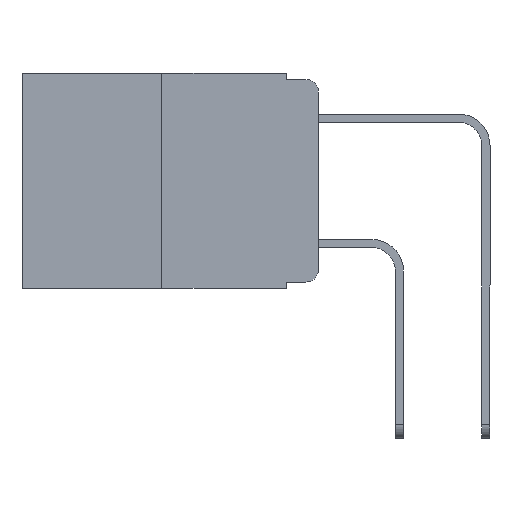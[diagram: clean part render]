
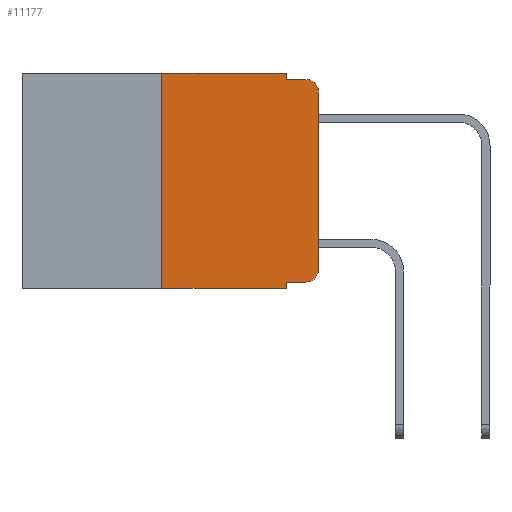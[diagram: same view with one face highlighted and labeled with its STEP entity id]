
A CAD part, left-side view. The second image highlights one B-rep face of the part: STEP entity #11177.
In plain terms, the highlighted planar face has unit normal (-1, 0, 0).
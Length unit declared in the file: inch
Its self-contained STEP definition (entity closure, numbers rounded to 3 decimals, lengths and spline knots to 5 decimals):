
#42 = VERTEX_POINT ( 'NONE', #2022 ) ;
#273 = CARTESIAN_POINT ( 'NONE',  ( 0., 0., 0. ) ) ;
#367 = LINE ( 'NONE', #6275, #9779 ) ;
#527 = CARTESIAN_POINT ( 'NONE',  ( 0., 0.02, -0.01 ) ) ;
#575 = VECTOR ( 'NONE', #2385, 39.37008 ) ;
#760 = CIRCLE ( 'NONE', #11905, 0.02 ) ;
#951 = VERTEX_POINT ( 'NONE', #1294 ) ;
#1268 = CARTESIAN_POINT ( 'NONE',  ( 0., 0.051, -0.333 ) ) ;
#1294 = CARTESIAN_POINT ( 'NONE',  ( 0., 0.25, -0.343 ) ) ;
#1402 = ORIENTED_EDGE ( 'NONE', *, *, #9388, .T. ) ;
#1609 = AXIS2_PLACEMENT_3D ( 'NONE', #4874, #11121, #5756 ) ;
#1796 = CARTESIAN_POINT ( 'NONE',  ( 0., 0., -0.313 ) ) ;
#1931 = ORIENTED_EDGE ( 'NONE', *, *, #2397, .T. ) ;
#1970 = CARTESIAN_POINT ( 'NONE',  ( 0., 0.473, 0. ) ) ;
#2022 = CARTESIAN_POINT ( 'NONE',  ( 0., 0.051, -0.01 ) ) ;
#2036 = LINE ( 'NONE', #2181, #11490 ) ;
#2161 = VERTEX_POINT ( 'NONE', #1268 ) ;
#2181 = CARTESIAN_POINT ( 'NONE',  ( 0., 0.051, -0.333 ) ) ;
#2385 = DIRECTION ( 'NONE',  ( 0., 0., 1. ) ) ;
#2397 = EDGE_CURVE ( 'NONE', #2161, #5680, #2036, .T. ) ;
#2660 = DIRECTION ( 'NONE',  ( 0., 0., -1. ) ) ;
#2750 = CARTESIAN_POINT ( 'NONE',  ( 0., 0.25, 0. ) ) ;
#2762 = CARTESIAN_POINT ( 'NONE',  ( 0., 0.051, -0.01 ) ) ;
#2780 = DIRECTION ( 'NONE',  ( 0., -1., 0. ) ) ;
#2800 = ORIENTED_EDGE ( 'NONE', *, *, #3113, .F. ) ;
#2962 = DIRECTION ( 'NONE',  ( 0., -1., 0. ) ) ;
#3113 = EDGE_CURVE ( 'NONE', #42, #8271, #11598, .T. ) ;
#3296 = VECTOR ( 'NONE', #2962, 39.37008 ) ;
#3611 = CARTESIAN_POINT ( 'NONE',  ( 0., 0.051, 0. ) ) ;
#3636 = LINE ( 'NONE', #3611, #10565 ) ;
#4311 = CARTESIAN_POINT ( 'NONE',  ( 0., 0.02, -0.313 ) ) ;
#4380 = DIRECTION ( 'NONE',  ( -1., 0., 0. ) ) ;
#4516 = VERTEX_POINT ( 'NONE', #6715 ) ;
#4738 = ORIENTED_EDGE ( 'NONE', *, *, #8730, .T. ) ;
#4758 = EDGE_CURVE ( 'NONE', #4993, #5213, #7643, .T. ) ;
#4874 = CARTESIAN_POINT ( 'NONE',  ( 0., 0.473, 0. ) ) ;
#4919 = CARTESIAN_POINT ( 'NONE',  ( 0., 0., -0.03 ) ) ;
#4993 = VERTEX_POINT ( 'NONE', #1796 ) ;
#5134 = ORIENTED_EDGE ( 'NONE', *, *, #9379, .F. ) ;
#5213 = VERTEX_POINT ( 'NONE', #4919 ) ;
#5244 = DIRECTION ( 'NONE',  ( 0., 0., -1. ) ) ;
#5267 = CARTESIAN_POINT ( 'NONE',  ( 0., 0.25, 0. ) ) ;
#5283 = VECTOR ( 'NONE', #7697, 39.37008 ) ;
#5497 = LINE ( 'NONE', #5267, #575 ) ;
#5576 = EDGE_CURVE ( 'NONE', #11036, #42, #3636, .T. ) ;
#5593 = ORIENTED_EDGE ( 'NONE', *, *, #4758, .T. ) ;
#5611 = FACE_OUTER_BOUND ( 'NONE', #11204, .T. ) ;
#5680 = VERTEX_POINT ( 'NONE', #6554 ) ;
#5756 = DIRECTION ( 'NONE',  ( 0., 0., -1. ) ) ;
#5774 = LINE ( 'NONE', #1970, #3296 ) ;
#5974 = EDGE_CURVE ( 'NONE', #951, #4516, #11000, .T. ) ;
#6271 = ORIENTED_EDGE ( 'NONE', *, *, #7440, .F. ) ;
#6275 = CARTESIAN_POINT ( 'NONE',  ( 0., 0.051, 0. ) ) ;
#6554 = CARTESIAN_POINT ( 'NONE',  ( 0., 0.02, -0.333 ) ) ;
#6715 = CARTESIAN_POINT ( 'NONE',  ( 0., 0.051, -0.343 ) ) ;
#6803 = VERTEX_POINT ( 'NONE', #2750 ) ;
#6968 = DIRECTION ( 'NONE',  ( 0., -1., 0. ) ) ;
#7173 = DIRECTION ( 'NONE',  ( 0., 0., -1. ) ) ;
#7440 = EDGE_CURVE ( 'NONE', #6803, #11036, #5774, .T. ) ;
#7636 = AXIS2_PLACEMENT_3D ( 'NONE', #9743, #4380, #10651 ) ;
#7643 = LINE ( 'NONE', #273, #5283 ) ;
#7697 = DIRECTION ( 'NONE',  ( 0., 0., 1. ) ) ;
#8271 = VERTEX_POINT ( 'NONE', #527 ) ;
#8412 = PLANE ( 'NONE',  #1609 ) ;
#8607 = VECTOR ( 'NONE', #6968, 39.37008 ) ;
#8644 = DIRECTION ( 'NONE',  ( 0., -1., 0. ) ) ;
#8654 = VECTOR ( 'NONE', #2780, 39.37008 ) ;
#8730 = EDGE_CURVE ( 'NONE', #5680, #4993, #760, .T. ) ;
#9056 = CARTESIAN_POINT ( 'NONE',  ( 0., 0.051, 0. ) ) ;
#9243 = ORIENTED_EDGE ( 'NONE', *, *, #11559, .F. ) ;
#9379 = EDGE_CURVE ( 'NONE', #951, #6803, #5497, .T. ) ;
#9388 = EDGE_CURVE ( 'NONE', #5213, #8271, #9963, .T. ) ;
#9743 = CARTESIAN_POINT ( 'NONE',  ( 0., 0.02, -0.03 ) ) ;
#9779 = VECTOR ( 'NONE', #7173, 39.37008 ) ;
#9797 = ORIENTED_EDGE ( 'NONE', *, *, #5576, .F. ) ;
#9963 = CIRCLE ( 'NONE', #7636, 0.02 ) ;
#10565 = VECTOR ( 'NONE', #2660, 39.37008 ) ;
#10586 = DIRECTION ( 'NONE',  ( -1., 0., 0. ) ) ;
#10651 = DIRECTION ( 'NONE',  ( 0., 0., -1. ) ) ;
#11000 = LINE ( 'NONE', #11459, #8607 ) ;
#11036 = VERTEX_POINT ( 'NONE', #9056 ) ;
#11121 = DIRECTION ( 'NONE',  ( 1., 0., 0. ) ) ;
#11177 = ADVANCED_FACE ( 'NONE', ( #5611 ), #8412, .F. ) ;
#11204 = EDGE_LOOP ( 'NONE', ( #5593, #1402, #2800, #9797, #6271, #5134, #11909, #9243, #1931, #4738 ) ) ;
#11459 = CARTESIAN_POINT ( 'NONE',  ( 0., 0.473, -0.343 ) ) ;
#11490 = VECTOR ( 'NONE', #8644, 39.37008 ) ;
#11559 = EDGE_CURVE ( 'NONE', #2161, #4516, #367, .T. ) ;
#11598 = LINE ( 'NONE', #2762, #8654 ) ;
#11905 = AXIS2_PLACEMENT_3D ( 'NONE', #4311, #10586, #5244 ) ;
#11909 = ORIENTED_EDGE ( 'NONE', *, *, #5974, .T. ) ;
